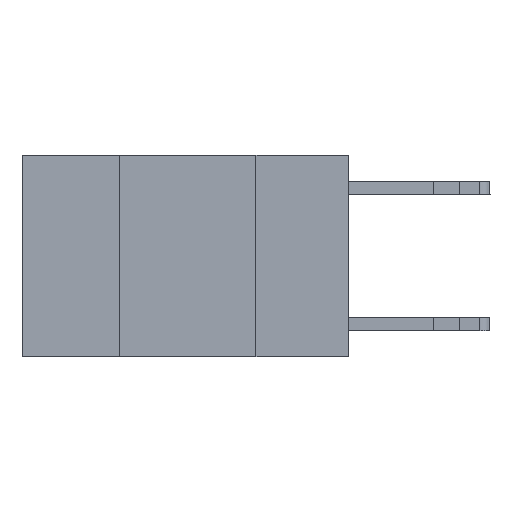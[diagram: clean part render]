
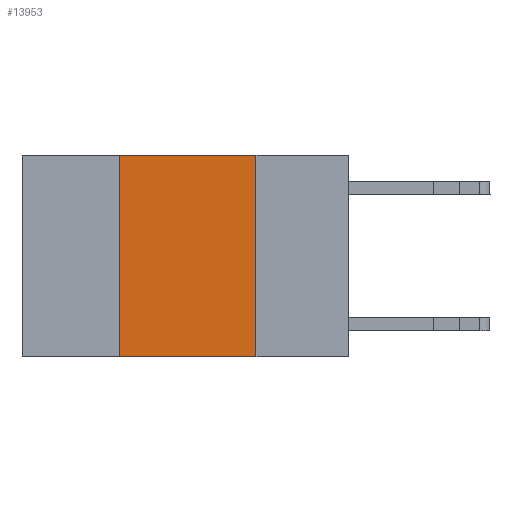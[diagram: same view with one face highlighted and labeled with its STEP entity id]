
A CAD part, left-side view. The second image highlights one B-rep face of the part: STEP entity #13953.
In plain terms, the highlighted planar face has unit normal (-1, 0, 0).
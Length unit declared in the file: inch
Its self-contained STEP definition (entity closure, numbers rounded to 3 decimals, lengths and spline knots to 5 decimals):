
#367 = VERTEX_POINT ( 'NONE', #12565 ) ;
#739 = DIRECTION ( 'NONE',  ( 1., 0., 0. ) ) ;
#1124 = VECTOR ( 'NONE', #15366, 39.37008 ) ;
#2667 = CARTESIAN_POINT ( 'NONE',  ( 0., 0.6, 0. ) ) ;
#2966 = LINE ( 'NONE', #16766, #9907 ) ;
#3305 = ORIENTED_EDGE ( 'NONE', *, *, #17823, .F. ) ;
#3679 = VECTOR ( 'NONE', #17169, 39.37008 ) ;
#3685 = PLANE ( 'NONE',  #15152 ) ;
#5110 = DIRECTION ( 'NONE',  ( 0., 0., 1. ) ) ;
#5190 = CARTESIAN_POINT ( 'NONE',  ( 0., 0.6, 0. ) ) ;
#5424 = CARTESIAN_POINT ( 'NONE',  ( 0., 0.17, 0. ) ) ;
#6305 = FACE_OUTER_BOUND ( 'NONE', #10894, .T. ) ;
#6710 = CARTESIAN_POINT ( 'NONE',  ( 0., 0.17, 0. ) ) ;
#7324 = LINE ( 'NONE', #13842, #7788 ) ;
#7788 = VECTOR ( 'NONE', #5110, 39.37008 ) ;
#8031 = VERTEX_POINT ( 'NONE', #17675 ) ;
#8481 = EDGE_CURVE ( 'NONE', #8031, #18001, #11536, .T. ) ;
#9225 = EDGE_CURVE ( 'NONE', #367, #15368, #2966, .T. ) ;
#9907 = VECTOR ( 'NONE', #12585, 39.37008 ) ;
#9940 = LINE ( 'NONE', #6710, #1124 ) ;
#10894 = EDGE_LOOP ( 'NONE', ( #14246, #16513, #3305, #18224 ) ) ;
#11124 = DIRECTION ( 'NONE',  ( 0., 0., -1. ) ) ;
#11536 = LINE ( 'NONE', #2667, #3679 ) ;
#12565 = CARTESIAN_POINT ( 'NONE',  ( 0., 0.42, -0.37 ) ) ;
#12585 = DIRECTION ( 'NONE',  ( 0., -1., 0. ) ) ;
#13842 = CARTESIAN_POINT ( 'NONE',  ( 0., 0.42, 0. ) ) ;
#13953 = ADVANCED_FACE ( 'NONE', ( #6305 ), #3685, .F. ) ;
#14246 = ORIENTED_EDGE ( 'NONE', *, *, #14979, .F. ) ;
#14979 = EDGE_CURVE ( 'NONE', #18001, #15368, #9940, .T. ) ;
#15152 = AXIS2_PLACEMENT_3D ( 'NONE', #5190, #739, #11124 ) ;
#15366 = DIRECTION ( 'NONE',  ( 0., 0., -1. ) ) ;
#15368 = VERTEX_POINT ( 'NONE', #17562 ) ;
#16513 = ORIENTED_EDGE ( 'NONE', *, *, #8481, .F. ) ;
#16766 = CARTESIAN_POINT ( 'NONE',  ( 0., 0.6, -0.37 ) ) ;
#17169 = DIRECTION ( 'NONE',  ( 0., -1., 0. ) ) ;
#17562 = CARTESIAN_POINT ( 'NONE',  ( 0., 0.17, -0.37 ) ) ;
#17675 = CARTESIAN_POINT ( 'NONE',  ( 0., 0.42, 0. ) ) ;
#17823 = EDGE_CURVE ( 'NONE', #367, #8031, #7324, .T. ) ;
#18001 = VERTEX_POINT ( 'NONE', #5424 ) ;
#18224 = ORIENTED_EDGE ( 'NONE', *, *, #9225, .T. ) ;
